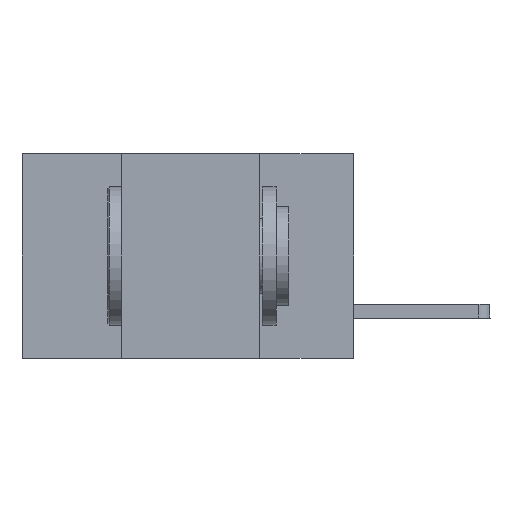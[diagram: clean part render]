
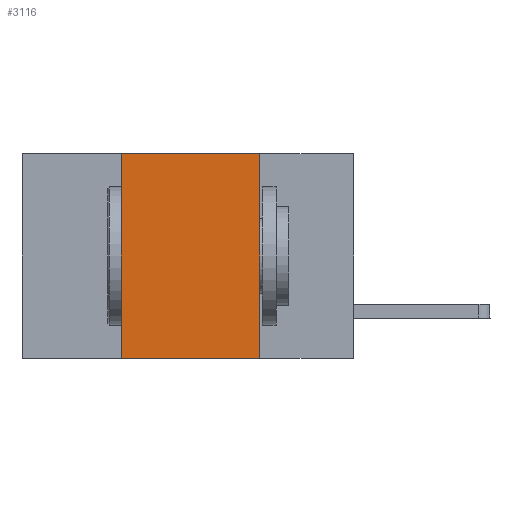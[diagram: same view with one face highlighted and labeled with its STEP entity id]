
A CAD part, left-side view. The second image highlights one B-rep face of the part: STEP entity #3116.
In plain terms, the highlighted planar face has unit normal (-1, 0, 0).
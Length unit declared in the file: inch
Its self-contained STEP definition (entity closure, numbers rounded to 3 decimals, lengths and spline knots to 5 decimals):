
#96 = VERTEX_POINT ( 'NONE', #2471 ) ;
#152 = VERTEX_POINT ( 'NONE', #5694 ) ;
#682 = VECTOR ( 'NONE', #2841, 39.37008 ) ;
#1938 = VECTOR ( 'NONE', #7536, 39.37008 ) ;
#2084 = VERTEX_POINT ( 'NONE', #8690 ) ;
#2471 = CARTESIAN_POINT ( 'NONE',  ( 0., 0.17, -0.37 ) ) ;
#2609 = ORIENTED_EDGE ( 'NONE', *, *, #7382, .T. ) ;
#2622 = DIRECTION ( 'NONE',  ( 0., 0., -1. ) ) ;
#2684 = ORIENTED_EDGE ( 'NONE', *, *, #4036, .F. ) ;
#2841 = DIRECTION ( 'NONE',  ( 0., -1., 0. ) ) ;
#3116 = ADVANCED_FACE ( 'NONE', ( #9450 ), #8265, .F. ) ;
#3406 = AXIS2_PLACEMENT_3D ( 'NONE', #5917, #7011, #13988 ) ;
#3426 = LINE ( 'NONE', #6025, #682 ) ;
#3438 = LINE ( 'NONE', #11034, #1938 ) ;
#4036 = EDGE_CURVE ( 'NONE', #2084, #13620, #3426, .T. ) ;
#4346 = CARTESIAN_POINT ( 'NONE',  ( 0., 0.6, -0.37 ) ) ;
#4608 = ORIENTED_EDGE ( 'NONE', *, *, #14723, .F. ) ;
#4812 = VECTOR ( 'NONE', #2622, 39.37008 ) ;
#5694 = CARTESIAN_POINT ( 'NONE',  ( 0., 0.42, -0.37 ) ) ;
#5917 = CARTESIAN_POINT ( 'NONE',  ( 0., 0.6, 0. ) ) ;
#6025 = CARTESIAN_POINT ( 'NONE',  ( 0., 0.6, 0. ) ) ;
#6076 = VECTOR ( 'NONE', #6724, 39.37008 ) ;
#6724 = DIRECTION ( 'NONE',  ( 0., -1., 0. ) ) ;
#6804 = LINE ( 'NONE', #4346, #6076 ) ;
#7011 = DIRECTION ( 'NONE',  ( 1., 0., 0. ) ) ;
#7382 = EDGE_CURVE ( 'NONE', #152, #96, #6804, .T. ) ;
#7436 = CARTESIAN_POINT ( 'NONE',  ( 0., 0.17, 0. ) ) ;
#7536 = DIRECTION ( 'NONE',  ( 0., 0., 1. ) ) ;
#8256 = ORIENTED_EDGE ( 'NONE', *, *, #11512, .F. ) ;
#8265 = PLANE ( 'NONE',  #3406 ) ;
#8393 = EDGE_LOOP ( 'NONE', ( #4608, #2684, #8256, #2609 ) ) ;
#8690 = CARTESIAN_POINT ( 'NONE',  ( 0., 0.42, 0. ) ) ;
#9450 = FACE_OUTER_BOUND ( 'NONE', #8393, .T. ) ;
#11034 = CARTESIAN_POINT ( 'NONE',  ( 0., 0.42, 0. ) ) ;
#11512 = EDGE_CURVE ( 'NONE', #152, #2084, #3438, .T. ) ;
#12748 = CARTESIAN_POINT ( 'NONE',  ( 0., 0.17, 0. ) ) ;
#13620 = VERTEX_POINT ( 'NONE', #7436 ) ;
#13988 = DIRECTION ( 'NONE',  ( 0., 0., -1. ) ) ;
#14723 = EDGE_CURVE ( 'NONE', #13620, #96, #14951, .T. ) ;
#14951 = LINE ( 'NONE', #12748, #4812 ) ;
